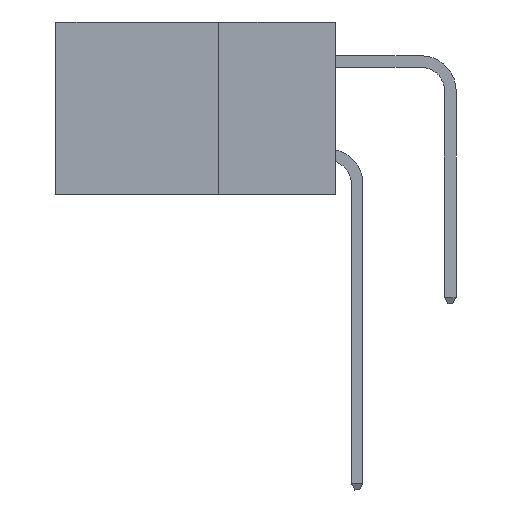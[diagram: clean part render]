
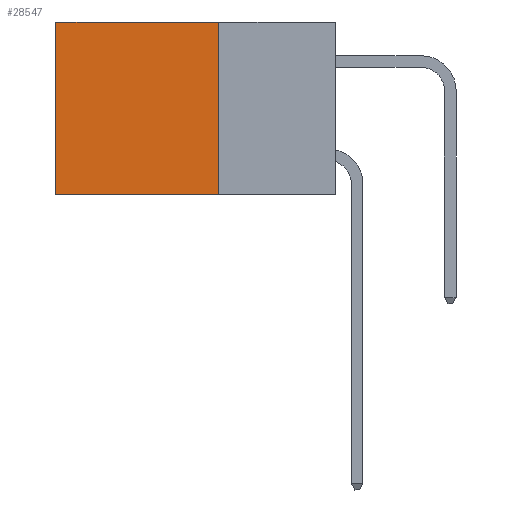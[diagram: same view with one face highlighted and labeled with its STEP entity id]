
A CAD part, left-side view. The second image highlights one B-rep face of the part: STEP entity #28547.
In plain terms, the highlighted planar face has unit normal (-1, 0, 0).
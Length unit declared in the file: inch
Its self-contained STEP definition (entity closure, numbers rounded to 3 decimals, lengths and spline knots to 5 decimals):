
#163 = LINE ( 'NONE', #5623, #547 ) ;
#533 = DIRECTION ( 'NONE',  ( 0., 1., 0. ) ) ;
#547 = VECTOR ( 'NONE', #533, 39.37008 ) ;
#3510 = DIRECTION ( 'NONE',  ( 0., 0., -1. ) ) ;
#3582 = LINE ( 'NONE', #16358, #19552 ) ;
#4902 = VERTEX_POINT ( 'NONE', #24065 ) ;
#5519 = VECTOR ( 'NONE', #21581, 39.37008 ) ;
#5623 = CARTESIAN_POINT ( 'NONE',  ( 0.2875, 0.25, 0. ) ) ;
#7264 = DIRECTION ( 'NONE',  ( 0., 1., 0. ) ) ;
#7352 = VERTEX_POINT ( 'NONE', #27592 ) ;
#7508 = ORIENTED_EDGE ( 'NONE', *, *, #10807, .T. ) ;
#10052 = CARTESIAN_POINT ( 'NONE',  ( 0.2875, 0.25, 0. ) ) ;
#10807 = EDGE_CURVE ( 'NONE', #7352, #4902, #15174, .T. ) ;
#13713 = VECTOR ( 'NONE', #19888, 39.37008 ) ;
#15052 = DIRECTION ( 'NONE',  ( 1., 0., 0. ) ) ;
#15089 = FACE_OUTER_BOUND ( 'NONE', #28434, .T. ) ;
#15174 = LINE ( 'NONE', #22366, #13713 ) ;
#16358 = CARTESIAN_POINT ( 'NONE',  ( 0.2875, 0.25, -0.37 ) ) ;
#19131 = CARTESIAN_POINT ( 'NONE',  ( 0.2875, 0.25, 0. ) ) ;
#19552 = VECTOR ( 'NONE', #7264, 39.37008 ) ;
#19888 = DIRECTION ( 'NONE',  ( 0., 0., -1. ) ) ;
#20949 = VERTEX_POINT ( 'NONE', #29625 ) ;
#21036 = EDGE_CURVE ( 'NONE', #20949, #7352, #163, .T. ) ;
#21581 = DIRECTION ( 'NONE',  ( 0., 0., -1. ) ) ;
#22366 = CARTESIAN_POINT ( 'NONE',  ( 0.2875, 0.6, 0. ) ) ;
#22447 = AXIS2_PLACEMENT_3D ( 'NONE', #10052, #15052, #3510 ) ;
#22819 = ORIENTED_EDGE ( 'NONE', *, *, #21036, .T. ) ;
#24065 = CARTESIAN_POINT ( 'NONE',  ( 0.2875, 0.6, -0.37 ) ) ;
#25477 = LINE ( 'NONE', #19131, #5519 ) ;
#25711 = EDGE_CURVE ( 'NONE', #20949, #26741, #25477, .T. ) ;
#26053 = ORIENTED_EDGE ( 'NONE', *, *, #25711, .F. ) ;
#26741 = VERTEX_POINT ( 'NONE', #27595 ) ;
#27092 = EDGE_CURVE ( 'NONE', #26741, #4902, #3582, .T. ) ;
#27358 = ORIENTED_EDGE ( 'NONE', *, *, #27092, .F. ) ;
#27592 = CARTESIAN_POINT ( 'NONE',  ( 0.2875, 0.6, 0. ) ) ;
#27595 = CARTESIAN_POINT ( 'NONE',  ( 0.2875, 0.25, -0.37 ) ) ;
#28434 = EDGE_LOOP ( 'NONE', ( #7508, #27358, #26053, #22819 ) ) ;
#28547 = ADVANCED_FACE ( 'NONE', ( #15089 ), #28687, .F. ) ;
#28687 = PLANE ( 'NONE',  #22447 ) ;
#29625 = CARTESIAN_POINT ( 'NONE',  ( 0.2875, 0.25, 0. ) ) ;
